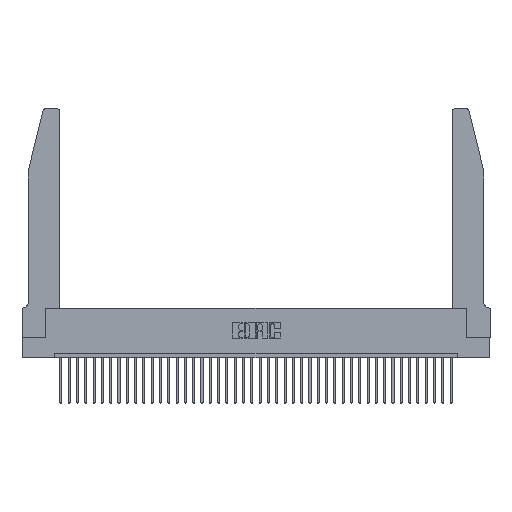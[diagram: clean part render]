
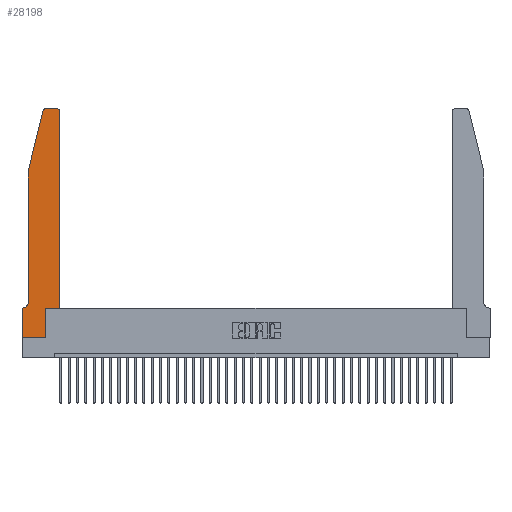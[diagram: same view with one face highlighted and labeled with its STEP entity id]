
A CAD part, top view. The second image highlights one B-rep face of the part: STEP entity #28198.
In plain terms, the highlighted planar face has unit normal (0, 0, 1).
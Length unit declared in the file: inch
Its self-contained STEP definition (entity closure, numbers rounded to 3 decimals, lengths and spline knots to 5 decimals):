
#708 = DIRECTION ( 'NONE',  ( 1., 0., 0. ) ) ;
#1374 = LINE ( 'NONE', #10185, #19241 ) ;
#1515 = CARTESIAN_POINT ( 'NONE',  ( 0.0055, 0.42, 0.37 ) ) ;
#1705 = VERTEX_POINT ( 'NONE', #7904 ) ;
#2470 = DIRECTION ( 'NONE',  ( 0., -1., 0. ) ) ;
#2480 = CARTESIAN_POINT ( 'NONE',  ( 0.2605, 2.75, 0.37 ) ) ;
#3045 = CARTESIAN_POINT ( 'NONE',  ( 0., 0.35, 0.37 ) ) ;
#3175 = EDGE_CURVE ( 'NONE', #37169, #35890, #27791, .T. ) ;
#3553 = CIRCLE ( 'NONE', #33526, 0.03 ) ;
#3941 = CARTESIAN_POINT ( 'NONE',  ( 0., 0.35, 0.37 ) ) ;
#4191 = LINE ( 'NONE', #29866, #36572 ) ;
#4204 = ORIENTED_EDGE ( 'NONE', *, *, #17049, .T. ) ;
#4211 = CARTESIAN_POINT ( 'NONE',  ( 0., 0., 0.37 ) ) ;
#4906 = VECTOR ( 'NONE', #40062, 39.37008 ) ;
#5080 = VECTOR ( 'NONE', #16049, 39.37008 ) ;
#5361 = CARTESIAN_POINT ( 'NONE',  ( 0.2865, 0., 0.37 ) ) ;
#6478 = CARTESIAN_POINT ( 'NONE',  ( 0.25487, 2.72718, 0.37 ) ) ;
#6678 = VERTEX_POINT ( 'NONE', #17815 ) ;
#6949 = CARTESIAN_POINT ( 'NONE',  ( 0.4205, 2.72, 0.37 ) ) ;
#7904 = CARTESIAN_POINT ( 'NONE',  ( 0.0755, 2., 0.37 ) ) ;
#7945 = DIRECTION ( 'NONE',  ( 0., 1., 0. ) ) ;
#8659 = ORIENTED_EDGE ( 'NONE', *, *, #11265, .T. ) ;
#8856 = PLANE ( 'NONE',  #34891 ) ;
#8914 = AXIS2_PLACEMENT_3D ( 'NONE', #1515, #36002, #11086 ) ;
#9010 = EDGE_CURVE ( 'NONE', #32142, #21155, #25495, .T. ) ;
#9136 = EDGE_LOOP ( 'NONE', ( #38650, #4204, #28939, #34325, #38768, #8659, #20459, #38188, #28415, #39826, #29949, #32679 ) ) ;
#9894 = VERTEX_POINT ( 'NONE', #3941 ) ;
#10185 = CARTESIAN_POINT ( 'NONE',  ( 0., 0., 0.37 ) ) ;
#10201 = VERTEX_POINT ( 'NONE', #10544 ) ;
#10544 = CARTESIAN_POINT ( 'NONE',  ( 0.4505, 2.72, 0.37 ) ) ;
#11086 = DIRECTION ( 'NONE',  ( -1., 0., 0. ) ) ;
#11265 = EDGE_CURVE ( 'NONE', #19655, #9894, #20987, .T. ) ;
#11333 = CIRCLE ( 'NONE', #8914, 0.07 ) ;
#11434 = LINE ( 'NONE', #12257, #24982 ) ;
#12070 = DIRECTION ( 'NONE',  ( 1., 0., 0. ) ) ;
#12257 = CARTESIAN_POINT ( 'NONE',  ( 0.0755, 2., 0.37 ) ) ;
#12414 = CARTESIAN_POINT ( 'NONE',  ( 0.0055, 0.35, 0.37 ) ) ;
#12943 = EDGE_CURVE ( 'NONE', #10201, #24472, #20328, .T. ) ;
#13703 = VECTOR ( 'NONE', #25932, 39.37008 ) ;
#15651 = FACE_OUTER_BOUND ( 'NONE', #9136, .T. ) ;
#15896 = DIRECTION ( 'NONE',  ( -0.239, -0.971, 0. ) ) ;
#16049 = DIRECTION ( 'NONE',  ( 1., 0., 0. ) ) ;
#16422 = DIRECTION ( 'NONE',  ( 0., -1., 0. ) ) ;
#17049 = EDGE_CURVE ( 'NONE', #25137, #23946, #3553, .T. ) ;
#17815 = CARTESIAN_POINT ( 'NONE',  ( 0.0755, 0.42, 0.37 ) ) ;
#17836 = CARTESIAN_POINT ( 'NONE',  ( 0.4505, 0.35, 0.37 ) ) ;
#19241 = VECTOR ( 'NONE', #16422, 39.37008 ) ;
#19655 = VERTEX_POINT ( 'NONE', #12414 ) ;
#20328 = CIRCLE ( 'NONE', #22225, 0.03 ) ;
#20459 = ORIENTED_EDGE ( 'NONE', *, *, #21600, .T. ) ;
#20889 = DIRECTION ( 'NONE',  ( 1., 0., 0. ) ) ;
#20987 = LINE ( 'NONE', #38209, #35060 ) ;
#21155 = VERTEX_POINT ( 'NONE', #39766 ) ;
#21600 = EDGE_CURVE ( 'NONE', #9894, #37169, #1374, .T. ) ;
#22015 = EDGE_CURVE ( 'NONE', #1705, #6678, #37634, .T. ) ;
#22103 = CARTESIAN_POINT ( 'NONE',  ( 0.284, 2.75, 0.37 ) ) ;
#22225 = AXIS2_PLACEMENT_3D ( 'NONE', #6949, #28175, #708 ) ;
#23946 = VERTEX_POINT ( 'NONE', #6478 ) ;
#24359 = EDGE_CURVE ( 'NONE', #21155, #10201, #26778, .T. ) ;
#24472 = VERTEX_POINT ( 'NONE', #33813 ) ;
#24680 = DIRECTION ( 'NONE',  ( 0., 0., 1. ) ) ;
#24982 = VECTOR ( 'NONE', #15896, 39.37008 ) ;
#25137 = VERTEX_POINT ( 'NONE', #22103 ) ;
#25495 = LINE ( 'NONE', #17836, #37133 ) ;
#25574 = CARTESIAN_POINT ( 'NONE',  ( 0.2865, 0.35, 0.37 ) ) ;
#25932 = DIRECTION ( 'NONE',  ( 0., 1., 0. ) ) ;
#26225 = EDGE_CURVE ( 'NONE', #24472, #25137, #36844, .T. ) ;
#26778 = LINE ( 'NONE', #32281, #13703 ) ;
#27161 = EDGE_CURVE ( 'NONE', #35890, #32142, #4191, .T. ) ;
#27791 = LINE ( 'NONE', #4211, #5080 ) ;
#28175 = DIRECTION ( 'NONE',  ( 0., 0., 1. ) ) ;
#28198 = ADVANCED_FACE ( 'NONE', ( #15651 ), #8856, .T. ) ;
#28415 = ORIENTED_EDGE ( 'NONE', *, *, #27161, .T. ) ;
#28939 = ORIENTED_EDGE ( 'NONE', *, *, #39854, .T. ) ;
#29284 = DIRECTION ( 'NONE',  ( -1., 0., 0. ) ) ;
#29737 = DIRECTION ( 'NONE',  ( 0., 0., 1. ) ) ;
#29866 = CARTESIAN_POINT ( 'NONE',  ( 0.2865, 0.35, 0.37 ) ) ;
#29949 = ORIENTED_EDGE ( 'NONE', *, *, #24359, .T. ) ;
#30881 = CARTESIAN_POINT ( 'NONE',  ( 0., 0., 0.37 ) ) ;
#31361 = VECTOR ( 'NONE', #2470, 39.37008 ) ;
#32142 = VERTEX_POINT ( 'NONE', #25574 ) ;
#32275 = DIRECTION ( 'NONE',  ( 1., 0., 0. ) ) ;
#32281 = CARTESIAN_POINT ( 'NONE',  ( 0.4505, 0.35, 0.37 ) ) ;
#32679 = ORIENTED_EDGE ( 'NONE', *, *, #12943, .T. ) ;
#33526 = AXIS2_PLACEMENT_3D ( 'NONE', #35945, #29737, #20889 ) ;
#33813 = CARTESIAN_POINT ( 'NONE',  ( 0.4205, 2.75, 0.37 ) ) ;
#34172 = EDGE_CURVE ( 'NONE', #6678, #19655, #11333, .T. ) ;
#34325 = ORIENTED_EDGE ( 'NONE', *, *, #22015, .T. ) ;
#34891 = AXIS2_PLACEMENT_3D ( 'NONE', #3045, #24680, #12070 ) ;
#35060 = VECTOR ( 'NONE', #29284, 39.37008 ) ;
#35890 = VERTEX_POINT ( 'NONE', #5361 ) ;
#35945 = CARTESIAN_POINT ( 'NONE',  ( 0.284, 2.72, 0.37 ) ) ;
#36002 = DIRECTION ( 'NONE',  ( 0., 0., -1. ) ) ;
#36572 = VECTOR ( 'NONE', #7945, 39.37008 ) ;
#36844 = LINE ( 'NONE', #2480, #4906 ) ;
#37133 = VECTOR ( 'NONE', #32275, 39.37008 ) ;
#37169 = VERTEX_POINT ( 'NONE', #30881 ) ;
#37634 = LINE ( 'NONE', #39514, #31361 ) ;
#38188 = ORIENTED_EDGE ( 'NONE', *, *, #3175, .T. ) ;
#38209 = CARTESIAN_POINT ( 'NONE',  ( 0.0755, 0.35, 0.37 ) ) ;
#38650 = ORIENTED_EDGE ( 'NONE', *, *, #26225, .T. ) ;
#38768 = ORIENTED_EDGE ( 'NONE', *, *, #34172, .T. ) ;
#39514 = CARTESIAN_POINT ( 'NONE',  ( 0.0755, 2., 0.37 ) ) ;
#39766 = CARTESIAN_POINT ( 'NONE',  ( 0.4505, 0.35, 0.37 ) ) ;
#39826 = ORIENTED_EDGE ( 'NONE', *, *, #9010, .T. ) ;
#39854 = EDGE_CURVE ( 'NONE', #23946, #1705, #11434, .T. ) ;
#40062 = DIRECTION ( 'NONE',  ( -1., 0., 0. ) ) ;
